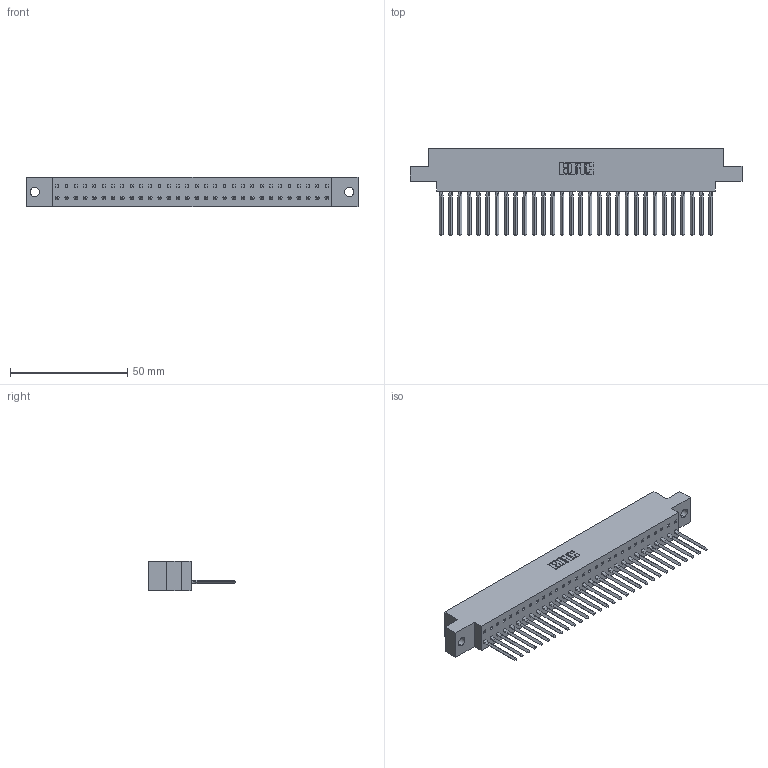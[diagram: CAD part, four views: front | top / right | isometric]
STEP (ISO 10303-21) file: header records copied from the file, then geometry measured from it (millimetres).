
FILE_DESCRIPTION (( 'STEP AP203' ), '1' );
FILE_NAME ('317-030-541-604.STEP', '2020-02-27T20:14:11', ( '' ), ( '' ), 'SwSTEP 2.0', 'SolidWorks 2016', '' );
FILE_SCHEMA (( 'CONFIG_CONTROL_DESIGN' ));
Length unit declared in the file: inch
Products named in the file (3): 317 Part_.156 Dia - TH; 317-290-002_541; 317-030-541-604
Assembly tree (31 placements, depth 2):
  317-030-541-604
    317 Part_.156 Dia - TH
    317-290-002_541  x30
Bounding box: 141.58 x 37.34 x 12.7 mm (x, y, z)
Volume: 22502.6 mm3; surface area: 31215.6 mm2
Topology: 31 solids, 31 shells, 4662 faces, 13295 edges, 8642 vertices
Faces by surface type: plane 3778, cylinder 764, bspline 120
Entity records: 45630 total; most frequent: CARTESIAN_POINT 8747, ORIENTED_EDGE 8030, DIRECTION 6587, EDGE_CURVE 4015, LINE 3651, VECTOR 3651, VERTEX_POINT 2668, AXIS2_PLACEMENT_3D 1468
